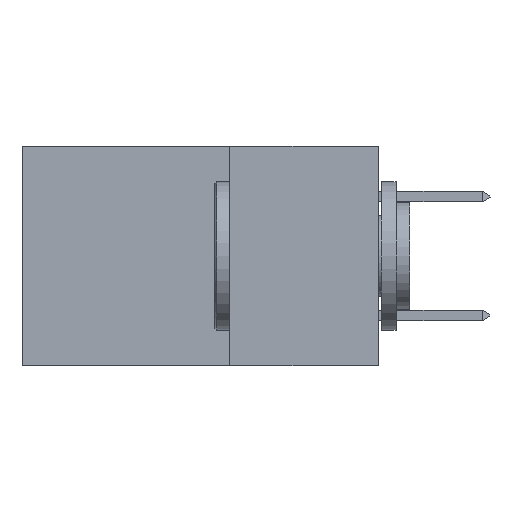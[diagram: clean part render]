
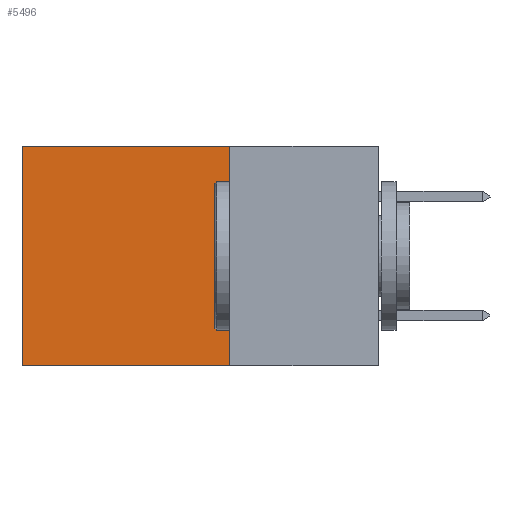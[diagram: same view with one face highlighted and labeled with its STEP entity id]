
A CAD part, left-side view. The second image highlights one B-rep face of the part: STEP entity #5496.
In plain terms, the highlighted planar face has unit normal (-1, 0, 0).
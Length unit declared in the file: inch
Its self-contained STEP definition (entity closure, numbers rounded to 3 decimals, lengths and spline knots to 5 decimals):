
#89 = LINE ( 'NONE', #333, #19558 ) ;
#333 = CARTESIAN_POINT ( 'NONE',  ( 0.298, 0.25, 0. ) ) ;
#545 = CARTESIAN_POINT ( 'NONE',  ( 0.298, 0.25, 0. ) ) ;
#703 = ORIENTED_EDGE ( 'NONE', *, *, #17945, .F. ) ;
#935 = ORIENTED_EDGE ( 'NONE', *, *, #22572, .T. ) ;
#1415 = AXIS2_PLACEMENT_3D ( 'NONE', #545, #2982, #20039 ) ;
#2914 = VECTOR ( 'NONE', #25326, 39.37008 ) ;
#2933 = VERTEX_POINT ( 'NONE', #7020 ) ;
#2982 = DIRECTION ( 'NONE',  ( 1., 0., 0. ) ) ;
#3548 = EDGE_CURVE ( 'NONE', #17335, #4745, #5684, .T. ) ;
#4745 = VERTEX_POINT ( 'NONE', #15035 ) ;
#4916 = VECTOR ( 'NONE', #30110, 39.37008 ) ;
#5496 = ADVANCED_FACE ( 'NONE', ( #27391 ), #10237, .F. ) ;
#5684 = LINE ( 'NONE', #17186, #4916 ) ;
#5885 = CARTESIAN_POINT ( 'NONE',  ( 0.298, 0.25, 0. ) ) ;
#7020 = CARTESIAN_POINT ( 'NONE',  ( 0.298, 0.25, 0. ) ) ;
#9327 = CARTESIAN_POINT ( 'NONE',  ( 0.298, 0.25, -0.37 ) ) ;
#10023 = DIRECTION ( 'NONE',  ( 0., 0., -1. ) ) ;
#10237 = PLANE ( 'NONE',  #1415 ) ;
#12592 = EDGE_CURVE ( 'NONE', #2933, #28287, #89, .T. ) ;
#14181 = DIRECTION ( 'NONE',  ( 0., 1., 0. ) ) ;
#14717 = ORIENTED_EDGE ( 'NONE', *, *, #12592, .F. ) ;
#15035 = CARTESIAN_POINT ( 'NONE',  ( 0.298, 0.6, -0.37 ) ) ;
#16952 = LINE ( 'NONE', #21337, #22583 ) ;
#17186 = CARTESIAN_POINT ( 'NONE',  ( 0.298, 0.6, 0. ) ) ;
#17335 = VERTEX_POINT ( 'NONE', #21157 ) ;
#17945 = EDGE_CURVE ( 'NONE', #28287, #4745, #16952, .T. ) ;
#19558 = VECTOR ( 'NONE', #10023, 39.37008 ) ;
#20039 = DIRECTION ( 'NONE',  ( 0., 0., -1. ) ) ;
#21157 = CARTESIAN_POINT ( 'NONE',  ( 0.298, 0.6, 0. ) ) ;
#21337 = CARTESIAN_POINT ( 'NONE',  ( 0.298, 0.25, -0.37 ) ) ;
#22572 = EDGE_CURVE ( 'NONE', #2933, #17335, #28759, .T. ) ;
#22583 = VECTOR ( 'NONE', #14181, 39.37008 ) ;
#25326 = DIRECTION ( 'NONE',  ( 0., 1., 0. ) ) ;
#27391 = FACE_OUTER_BOUND ( 'NONE', #28627, .T. ) ;
#27698 = ORIENTED_EDGE ( 'NONE', *, *, #3548, .T. ) ;
#28287 = VERTEX_POINT ( 'NONE', #9327 ) ;
#28627 = EDGE_LOOP ( 'NONE', ( #27698, #703, #14717, #935 ) ) ;
#28759 = LINE ( 'NONE', #5885, #2914 ) ;
#30110 = DIRECTION ( 'NONE',  ( 0., 0., -1. ) ) ;
